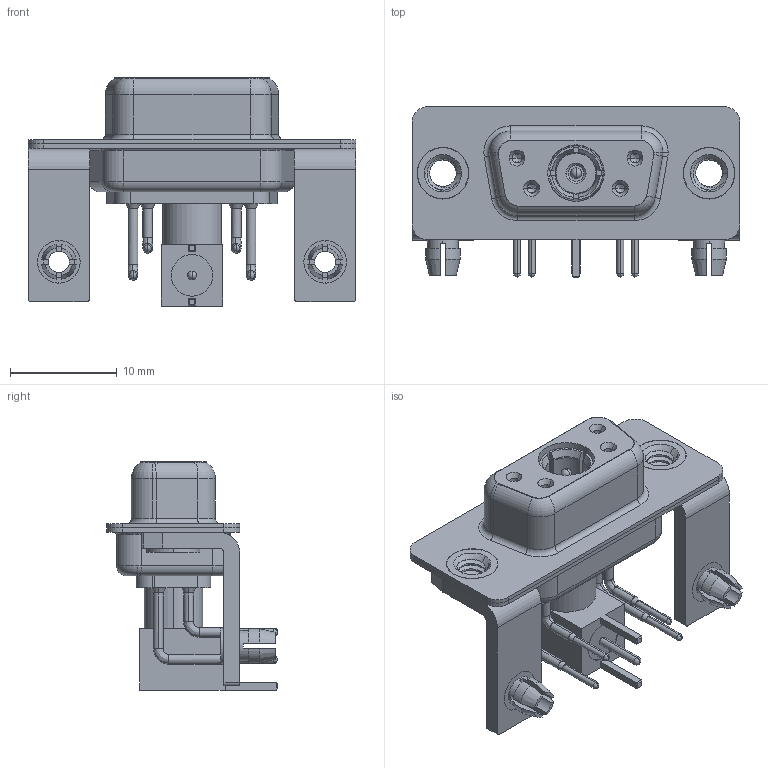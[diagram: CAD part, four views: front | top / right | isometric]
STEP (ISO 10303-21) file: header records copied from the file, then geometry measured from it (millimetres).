
FILE_DESCRIPTION (( 'STEP AP203' ), '1' );
FILE_NAME ('630-5W1-640-7TB.STEP', '2022-05-27T12:25:21', ( '' ), ( '' ), 'SwSTEP 2.0', 'SolidWorks 2020', '' );
FILE_SCHEMA (( 'CONFIG_CONTROL_DESIGN' ));
Length unit declared in the file: millimetre
Products named in the file (16): 630Combo Board Lock; 630Combo Contact Row 2; Insulator Pin_Straight PC Tail; 630-5W1-640-7TB; Co-Ax Plug Assy_RA; Insulator RA Pin; Pin_RA; Co-Ax Plug_RA PC Tail; 630Combo Housing_5W1; 630Combo Shell Rear_09 Contacts; RA Back Shell; 630Combo Contact Row 1; 630Combo Stabilizer Bracket; 630Combo Threaded Rivet_B; 630Combo Shell Front_09 Contacts; Locking Collar
Assembly tree (20 placements, depth 3):
  630-5W1-640-7TB
    630Combo Housing_5W1
    630Combo Shell Front_09 Contacts
    630Combo Shell Rear_09 Contacts
    630Combo Threaded Rivet_B  x2
    630Combo Stabilizer Bracket  x2
    630Combo Board Lock  x2
    Co-Ax Plug Assy_RA
      Co-Ax Plug_RA PC Tail
      Insulator Pin_Straight PC Tail
      Pin_RA
      Locking Collar
      RA Back Shell
      Insulator RA Pin
    630Combo Contact Row 1  x2
    630Combo Contact Row 2  x2
Bounding box: 30.8 x 16 x 21.41 mm (x, y, z)
Volume: 2269.5 mm3; surface area: 5810.1 mm2
Topology: 19 solids, 19 shells, 789 faces, 1970 edges, 1244 vertices
Faces by surface type: cylinder 344, plane 262, cone 93, torus 63, bspline 23, sphere 4
Entity records: 21732 total; most frequent: CARTESIAN_POINT 5120, DIRECTION 3321, ORIENTED_EDGE 2966, EDGE_CURVE 1483, AXIS2_PLACEMENT_3D 1334, VERTEX_POINT 943, CIRCLE 711, EDGE_LOOP 692
